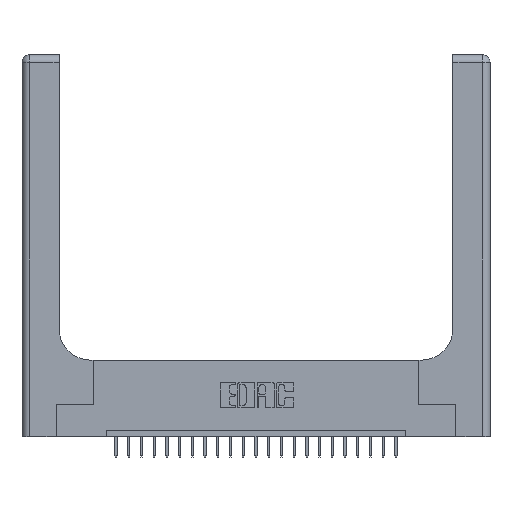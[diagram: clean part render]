
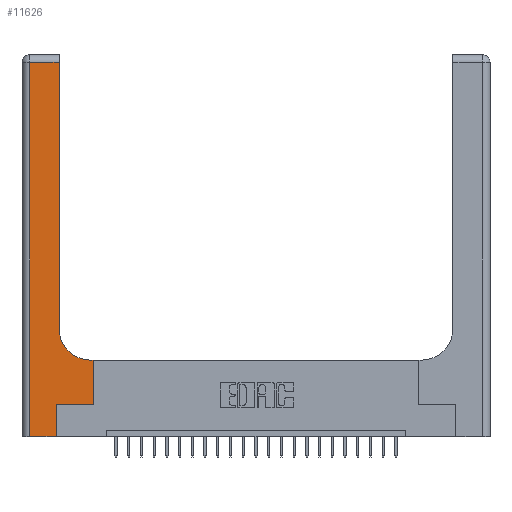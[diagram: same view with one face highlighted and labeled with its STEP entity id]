
A CAD part, top view. The second image highlights one B-rep face of the part: STEP entity #11626.
In plain terms, the highlighted planar face has unit normal (0, 0, 1).
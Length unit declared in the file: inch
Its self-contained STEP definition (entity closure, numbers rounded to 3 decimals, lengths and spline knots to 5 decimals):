
#867 = CARTESIAN_POINT ( 'NONE',  ( 0.2915, 3., 0.37 ) ) ;
#868 = CARTESIAN_POINT ( 'NONE',  ( 0.2915, 0.85, 0.37 ) ) ;
#1890 = FACE_OUTER_BOUND ( 'NONE', #6370, .T. ) ;
#2355 = VECTOR ( 'NONE', #3114, 39.37008 ) ;
#2481 = LINE ( 'NONE', #21268, #17445 ) ;
#2632 = CARTESIAN_POINT ( 'NONE',  ( 0.5585, 0.25, 0.37 ) ) ;
#3058 = DIRECTION ( 'NONE',  ( 0., 1., 0. ) ) ;
#3114 = DIRECTION ( 'NONE',  ( 1., 0., 0. ) ) ;
#4649 = DIRECTION ( 'NONE',  ( 0., 1., 0. ) ) ;
#4877 = LINE ( 'NONE', #10234, #19220 ) ;
#5718 = ORIENTED_EDGE ( 'NONE', *, *, #10261, .T. ) ;
#5983 = VERTEX_POINT ( 'NONE', #6107 ) ;
#6107 = CARTESIAN_POINT ( 'NONE',  ( 0.06, 2.94, 0.37 ) ) ;
#6366 = EDGE_CURVE ( 'NONE', #10326, #22386, #14209, .T. ) ;
#6370 = EDGE_LOOP ( 'NONE', ( #5718, #15196, #17611, #18774, #6890, #22543, #19628, #18637, #13147 ) ) ;
#6380 = EDGE_CURVE ( 'NONE', #9822, #24472, #24495, .T. ) ;
#6890 = ORIENTED_EDGE ( 'NONE', *, *, #13112, .T. ) ;
#8601 = VERTEX_POINT ( 'NONE', #17964 ) ;
#8911 = VERTEX_POINT ( 'NONE', #14412 ) ;
#9100 = VECTOR ( 'NONE', #4649, 39.37008 ) ;
#9123 = VECTOR ( 'NONE', #17226, 39.37008 ) ;
#9509 = CARTESIAN_POINT ( 'NONE',  ( 0.269, 0., 0.37 ) ) ;
#9542 = EDGE_CURVE ( 'NONE', #5983, #10653, #24299, .T. ) ;
#9822 = VERTEX_POINT ( 'NONE', #13975 ) ;
#9983 = CARTESIAN_POINT ( 'NONE',  ( 0.2915, 2.94, 0.37 ) ) ;
#10234 = CARTESIAN_POINT ( 'NONE',  ( 0.2915, 0.6, 0.37 ) ) ;
#10261 = EDGE_CURVE ( 'NONE', #22386, #23528, #16199, .T. ) ;
#10326 = VERTEX_POINT ( 'NONE', #16515 ) ;
#10653 = VERTEX_POINT ( 'NONE', #13743 ) ;
#11364 = CARTESIAN_POINT ( 'NONE',  ( 0., 3., 0.37 ) ) ;
#11626 = ADVANCED_FACE ( 'NONE', ( #1890 ), #23312, .F. ) ;
#11641 = AXIS2_PLACEMENT_3D ( 'NONE', #12628, #18504, #20424 ) ;
#12389 = DIRECTION ( 'NONE',  ( 1., 0., 0. ) ) ;
#12537 = DIRECTION ( 'NONE',  ( -1., 0., 0. ) ) ;
#12628 = CARTESIAN_POINT ( 'NONE',  ( 0.5415, 0.85, 0.37 ) ) ;
#13112 = EDGE_CURVE ( 'NONE', #8601, #9822, #17684, .T. ) ;
#13147 = ORIENTED_EDGE ( 'NONE', *, *, #6366, .T. ) ;
#13578 = DIRECTION ( 'NONE',  ( -1., 0., 0. ) ) ;
#13743 = CARTESIAN_POINT ( 'NONE',  ( 0.06, 0., 0.37 ) ) ;
#13975 = CARTESIAN_POINT ( 'NONE',  ( 0.269, 0.25, 0.37 ) ) ;
#14209 = CIRCLE ( 'NONE', #11641, 0.25 ) ;
#14412 = CARTESIAN_POINT ( 'NONE',  ( 0.5585, 0.6, 0.37 ) ) ;
#14895 = LINE ( 'NONE', #2632, #9100 ) ;
#15196 = ORIENTED_EDGE ( 'NONE', *, *, #21260, .T. ) ;
#15218 = CARTESIAN_POINT ( 'NONE',  ( 0.5585, 0.25, 0.37 ) ) ;
#15549 = DIRECTION ( 'NONE',  ( 0., 0., -1. ) ) ;
#16199 = LINE ( 'NONE', #867, #21597 ) ;
#16515 = CARTESIAN_POINT ( 'NONE',  ( 0.5415, 0.6, 0.37 ) ) ;
#16540 = DIRECTION ( 'NONE',  ( 0., -1., 0. ) ) ;
#16784 = CARTESIAN_POINT ( 'NONE',  ( 0., 0., 0.37 ) ) ;
#17226 = DIRECTION ( 'NONE',  ( 0., 1., 0. ) ) ;
#17445 = VECTOR ( 'NONE', #19411, 39.37008 ) ;
#17611 = ORIENTED_EDGE ( 'NONE', *, *, #9542, .T. ) ;
#17684 = LINE ( 'NONE', #9509, #9123 ) ;
#17964 = CARTESIAN_POINT ( 'NONE',  ( 0.269, 0., 0.37 ) ) ;
#18192 = VECTOR ( 'NONE', #12389, 39.37008 ) ;
#18504 = DIRECTION ( 'NONE',  ( 0., 0., -1. ) ) ;
#18593 = VECTOR ( 'NONE', #16540, 39.37008 ) ;
#18637 = ORIENTED_EDGE ( 'NONE', *, *, #20743, .T. ) ;
#18774 = ORIENTED_EDGE ( 'NONE', *, *, #23057, .T. ) ;
#19220 = VECTOR ( 'NONE', #12537, 39.37008 ) ;
#19411 = DIRECTION ( 'NONE',  ( -1., 0., 0. ) ) ;
#19628 = ORIENTED_EDGE ( 'NONE', *, *, #22310, .T. ) ;
#19867 = AXIS2_PLACEMENT_3D ( 'NONE', #11364, #15549, #13578 ) ;
#20424 = DIRECTION ( 'NONE',  ( 1., 0., 0. ) ) ;
#20743 = EDGE_CURVE ( 'NONE', #8911, #10326, #4877, .T. ) ;
#21260 = EDGE_CURVE ( 'NONE', #23528, #5983, #2481, .T. ) ;
#21268 = CARTESIAN_POINT ( 'NONE',  ( 0., 2.94, 0.37 ) ) ;
#21597 = VECTOR ( 'NONE', #3058, 39.37008 ) ;
#22310 = EDGE_CURVE ( 'NONE', #24472, #8911, #14895, .T. ) ;
#22344 = CARTESIAN_POINT ( 'NONE',  ( 0.06, 3., 0.37 ) ) ;
#22386 = VERTEX_POINT ( 'NONE', #868 ) ;
#22543 = ORIENTED_EDGE ( 'NONE', *, *, #6380, .T. ) ;
#23057 = EDGE_CURVE ( 'NONE', #10653, #8601, #24844, .T. ) ;
#23312 = PLANE ( 'NONE',  #19867 ) ;
#23528 = VERTEX_POINT ( 'NONE', #9983 ) ;
#23988 = CARTESIAN_POINT ( 'NONE',  ( 0.269, 0.25, 0.37 ) ) ;
#24299 = LINE ( 'NONE', #22344, #18593 ) ;
#24472 = VERTEX_POINT ( 'NONE', #15218 ) ;
#24495 = LINE ( 'NONE', #23988, #18192 ) ;
#24844 = LINE ( 'NONE', #16784, #2355 ) ;
